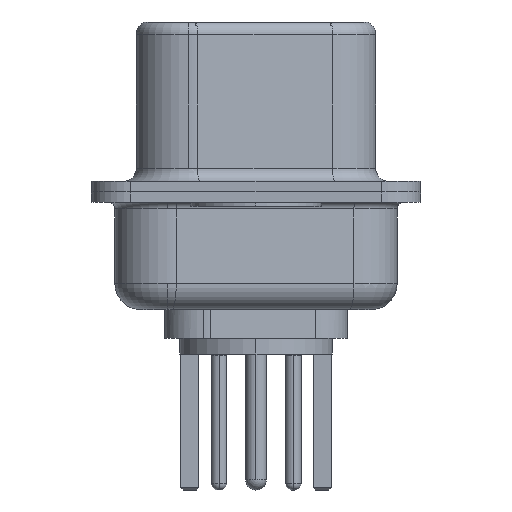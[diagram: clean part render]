
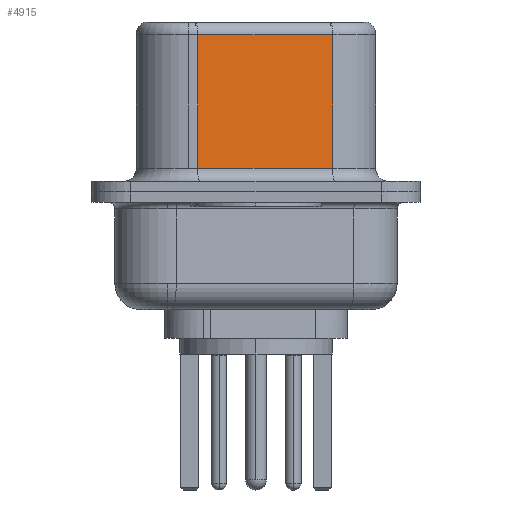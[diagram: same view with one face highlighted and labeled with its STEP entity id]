
A CAD part, left-side view. The second image highlights one B-rep face of the part: STEP entity #4915.
In plain terms, the highlighted planar face has unit normal (-0.985, -0.174, 0).
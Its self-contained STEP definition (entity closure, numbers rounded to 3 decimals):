
#305 = VECTOR ( 'NONE', #3492, 1000. ) ;
#652 = CARTESIAN_POINT ( 'NONE',  ( 4.58, -2.927, 6.52 ) ) ;
#666 = ORIENTED_EDGE ( 'NONE', *, *, #9496, .F. ) ;
#802 = LINE ( 'NONE', #6626, #305 ) ;
#1397 = CARTESIAN_POINT ( 'NONE',  ( 3.67, 2.233, 6.02 ) ) ;
#1571 = DIRECTION ( 'NONE',  ( 0., 0., -1. ) ) ;
#2319 = DIRECTION ( 'NONE',  ( 0.985, 0.174, 0. ) ) ;
#2403 = FACE_OUTER_BOUND ( 'NONE', #14923, .T. ) ;
#2644 = CARTESIAN_POINT ( 'NONE',  ( 3.67, 2.233, 0.9 ) ) ;
#2647 = EDGE_CURVE ( 'NONE', #9135, #19411, #19787, .T. ) ;
#3492 = DIRECTION ( 'NONE',  ( 0., 0., -1. ) ) ;
#3784 = VECTOR ( 'NONE', #14594, 1000. ) ;
#4915 = ADVANCED_FACE ( 'NONE', ( #2403 ), #16823, .F. ) ;
#5328 = DIRECTION ( 'NONE',  ( -0.174, 0.985, 0. ) ) ;
#6063 = LINE ( 'NONE', #652, #17782 ) ;
#6626 = CARTESIAN_POINT ( 'NONE',  ( 3.67, 2.233, 6.52 ) ) ;
#7271 = EDGE_CURVE ( 'NONE', #19411, #13688, #802, .T. ) ;
#7568 = VECTOR ( 'NONE', #11796, 1000. ) ;
#7909 = LINE ( 'NONE', #13039, #3784 ) ;
#8774 = VERTEX_POINT ( 'NONE', #15360 ) ;
#9135 = VERTEX_POINT ( 'NONE', #9225 ) ;
#9225 = CARTESIAN_POINT ( 'NONE',  ( 4.58, -2.927, 6.02 ) ) ;
#9496 = EDGE_CURVE ( 'NONE', #9135, #8774, #6063, .T. ) ;
#10249 = ORIENTED_EDGE ( 'NONE', *, *, #7271, .T. ) ;
#10713 = AXIS2_PLACEMENT_3D ( 'NONE', #11449, #2319, #5328 ) ;
#11449 = CARTESIAN_POINT ( 'NONE',  ( 4.58, -2.927, 6.52 ) ) ;
#11616 = ORIENTED_EDGE ( 'NONE', *, *, #2647, .T. ) ;
#11741 = CARTESIAN_POINT ( 'NONE',  ( 4.58, -2.927, 6.02 ) ) ;
#11796 = DIRECTION ( 'NONE',  ( -0.174, 0.985, 0. ) ) ;
#12549 = EDGE_CURVE ( 'NONE', #13688, #8774, #7909, .T. ) ;
#13039 = CARTESIAN_POINT ( 'NONE',  ( 4.58, -2.927, 0.9 ) ) ;
#13688 = VERTEX_POINT ( 'NONE', #2644 ) ;
#14594 = DIRECTION ( 'NONE',  ( 0.174, -0.985, 0. ) ) ;
#14923 = EDGE_LOOP ( 'NONE', ( #666, #11616, #10249, #16976 ) ) ;
#15360 = CARTESIAN_POINT ( 'NONE',  ( 4.58, -2.927, 0.9 ) ) ;
#16823 = PLANE ( 'NONE',  #10713 ) ;
#16976 = ORIENTED_EDGE ( 'NONE', *, *, #12549, .T. ) ;
#17782 = VECTOR ( 'NONE', #1571, 1000. ) ;
#19411 = VERTEX_POINT ( 'NONE', #1397 ) ;
#19787 = LINE ( 'NONE', #11741, #7568 ) ;
